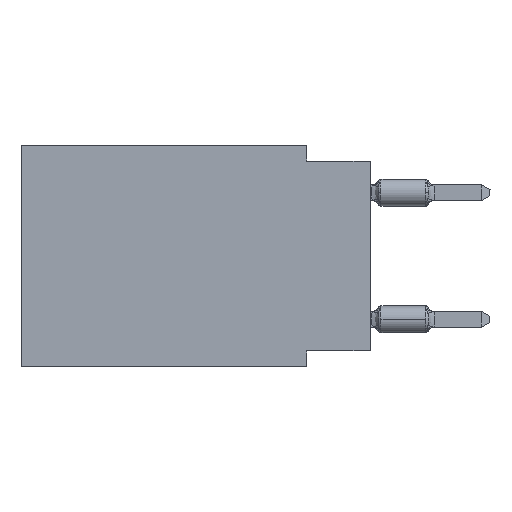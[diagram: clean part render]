
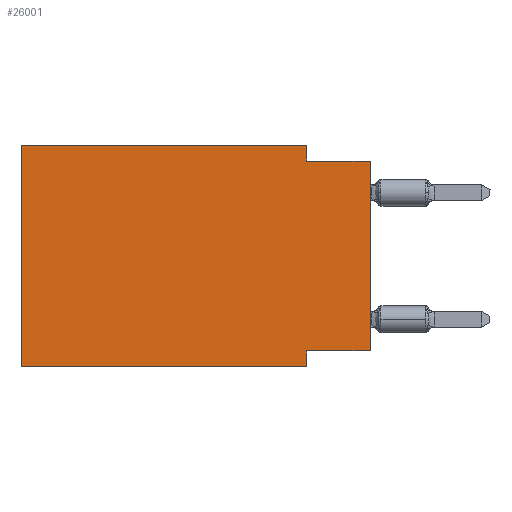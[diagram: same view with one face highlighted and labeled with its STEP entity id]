
A CAD part, left-side view. The second image highlights one B-rep face of the part: STEP entity #26001.
In plain terms, the highlighted planar face has unit normal (-1, 0, 0).
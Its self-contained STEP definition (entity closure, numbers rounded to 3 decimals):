
#362 = DIRECTION ( 'NONE',  ( 0., 1., 0. ) ) ;
#740 = LINE ( 'NONE', #24727, #18431 ) ;
#915 = VECTOR ( 'NONE', #24862, 1000. ) ;
#1221 = LINE ( 'NONE', #13304, #30607 ) ;
#1267 = CARTESIAN_POINT ( 'NONE',  ( 0., 13.97, 0. ) ) ;
#1603 = ORIENTED_EDGE ( 'NONE', *, *, #17109, .F. ) ;
#1680 = VECTOR ( 'NONE', #21485, 1000. ) ;
#1788 = CARTESIAN_POINT ( 'NONE',  ( 0., 0., -0.635 ) ) ;
#2291 = CARTESIAN_POINT ( 'NONE',  ( 0., 2.54, -8.89 ) ) ;
#2851 = VERTEX_POINT ( 'NONE', #1788 ) ;
#3465 = CARTESIAN_POINT ( 'NONE',  ( 0., 0., 0. ) ) ;
#3635 = ORIENTED_EDGE ( 'NONE', *, *, #33450, .F. ) ;
#3808 = CARTESIAN_POINT ( 'NONE',  ( 0., 13.97, -8.89 ) ) ;
#4205 = CARTESIAN_POINT ( 'NONE',  ( 0., 2.54, 0. ) ) ;
#5285 = EDGE_CURVE ( 'NONE', #6677, #23135, #1221, .T. ) ;
#6265 = FACE_OUTER_BOUND ( 'NONE', #8609, .T. ) ;
#6677 = VERTEX_POINT ( 'NONE', #4205 ) ;
#6846 = LINE ( 'NONE', #3465, #1680 ) ;
#8271 = ORIENTED_EDGE ( 'NONE', *, *, #5285, .F. ) ;
#8345 = CARTESIAN_POINT ( 'NONE',  ( 0., 2.54, -8.255 ) ) ;
#8609 = EDGE_LOOP ( 'NONE', ( #26813, #11191, #8271, #36831, #13613, #37499, #1603, #3635 ) ) ;
#9019 = DIRECTION ( 'NONE',  ( 0., -1., 0. ) ) ;
#9327 = VERTEX_POINT ( 'NONE', #8345 ) ;
#9995 = CARTESIAN_POINT ( 'NONE',  ( 0., 13.97, 0. ) ) ;
#11191 = ORIENTED_EDGE ( 'NONE', *, *, #23421, .F. ) ;
#12445 = CARTESIAN_POINT ( 'NONE',  ( 0., 13.97, -8.89 ) ) ;
#12652 = EDGE_CURVE ( 'NONE', #34390, #27483, #12761, .T. ) ;
#12761 = LINE ( 'NONE', #9995, #915 ) ;
#13304 = CARTESIAN_POINT ( 'NONE',  ( 0., 2.54, 0. ) ) ;
#13613 = ORIENTED_EDGE ( 'NONE', *, *, #12652, .F. ) ;
#14172 = VECTOR ( 'NONE', #32986, 1000. ) ;
#14737 = VERTEX_POINT ( 'NONE', #35195 ) ;
#14747 = LINE ( 'NONE', #17916, #14172 ) ;
#15855 = VECTOR ( 'NONE', #9019, 1000. ) ;
#15943 = CARTESIAN_POINT ( 'NONE',  ( 0., 2.54, -0.635 ) ) ;
#16350 = DIRECTION ( 'NONE',  ( 0., 0., -1. ) ) ;
#17109 = EDGE_CURVE ( 'NONE', #9327, #14737, #24619, .T. ) ;
#17916 = CARTESIAN_POINT ( 'NONE',  ( 0., 0., -0.635 ) ) ;
#18125 = LINE ( 'NONE', #27834, #15855 ) ;
#18431 = VECTOR ( 'NONE', #362, 1000. ) ;
#21485 = DIRECTION ( 'NONE',  ( 0., 0., 1. ) ) ;
#21807 = CARTESIAN_POINT ( 'NONE',  ( 0., 0., -8.255 ) ) ;
#23006 = VECTOR ( 'NONE', #25312, 1000. ) ;
#23135 = VERTEX_POINT ( 'NONE', #15943 ) ;
#23286 = DIRECTION ( 'NONE',  ( 0., 0., -1. ) ) ;
#23421 = EDGE_CURVE ( 'NONE', #23135, #2851, #14747, .T. ) ;
#24270 = EDGE_CURVE ( 'NONE', #34390, #14737, #27701, .T. ) ;
#24619 = LINE ( 'NONE', #2291, #30661 ) ;
#24727 = CARTESIAN_POINT ( 'NONE',  ( 0., 0., -8.255 ) ) ;
#24862 = DIRECTION ( 'NONE',  ( 0., 0., 1. ) ) ;
#25312 = DIRECTION ( 'NONE',  ( 0., -1., 0. ) ) ;
#25410 = DIRECTION ( 'NONE',  ( 0., 0., -1. ) ) ;
#26001 = ADVANCED_FACE ( 'NONE', ( #6265 ), #28635, .F. ) ;
#26813 = ORIENTED_EDGE ( 'NONE', *, *, #27315, .T. ) ;
#27315 = EDGE_CURVE ( 'NONE', #29506, #2851, #6846, .T. ) ;
#27483 = VERTEX_POINT ( 'NONE', #1267 ) ;
#27701 = LINE ( 'NONE', #12445, #23006 ) ;
#27834 = CARTESIAN_POINT ( 'NONE',  ( 0., 13.97, 0. ) ) ;
#28050 = DIRECTION ( 'NONE',  ( 1., 0., 0. ) ) ;
#28635 = PLANE ( 'NONE',  #30703 ) ;
#29506 = VERTEX_POINT ( 'NONE', #21807 ) ;
#30607 = VECTOR ( 'NONE', #25410, 1000. ) ;
#30661 = VECTOR ( 'NONE', #23286, 1000. ) ;
#30703 = AXIS2_PLACEMENT_3D ( 'NONE', #34382, #28050, #16350 ) ;
#32541 = EDGE_CURVE ( 'NONE', #27483, #6677, #18125, .T. ) ;
#32986 = DIRECTION ( 'NONE',  ( 0., -1., 0. ) ) ;
#33450 = EDGE_CURVE ( 'NONE', #29506, #9327, #740, .T. ) ;
#34382 = CARTESIAN_POINT ( 'NONE',  ( 0., 13.97, 0. ) ) ;
#34390 = VERTEX_POINT ( 'NONE', #3808 ) ;
#35195 = CARTESIAN_POINT ( 'NONE',  ( 0., 2.54, -8.89 ) ) ;
#36831 = ORIENTED_EDGE ( 'NONE', *, *, #32541, .F. ) ;
#37499 = ORIENTED_EDGE ( 'NONE', *, *, #24270, .T. ) ;
